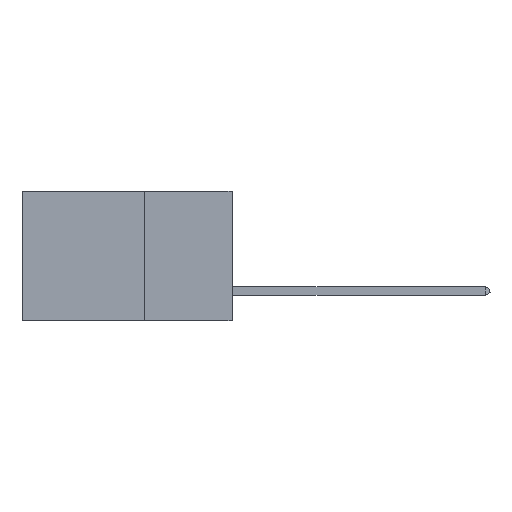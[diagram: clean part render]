
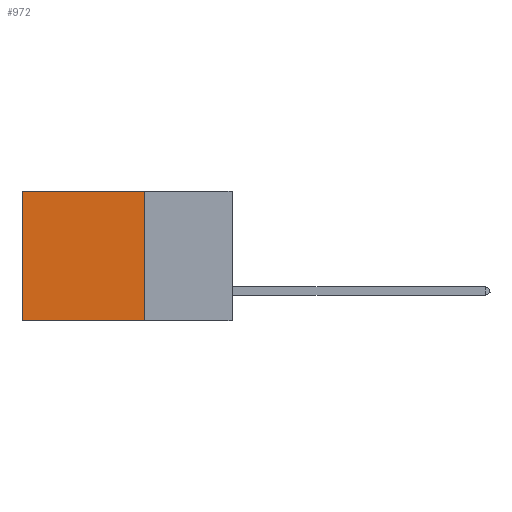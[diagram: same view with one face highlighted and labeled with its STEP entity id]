
A CAD part, left-side view. The second image highlights one B-rep face of the part: STEP entity #972.
In plain terms, the highlighted planar face has unit normal (-1, 0, 0).
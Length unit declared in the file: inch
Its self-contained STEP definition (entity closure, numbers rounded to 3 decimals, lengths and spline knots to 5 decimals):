
#972 = ADVANCED_FACE ( 'NONE', ( #11237 ), #6562, .F. ) ;
#2594 = VERTEX_POINT ( 'NONE', #11656 ) ;
#3535 = EDGE_CURVE ( 'NONE', #2594, #25100, #17388, .T. ) ;
#3725 = DIRECTION ( 'NONE',  ( 0., 1., 0. ) ) ;
#4094 = VECTOR ( 'NONE', #16937, 39.37008 ) ;
#5048 = CARTESIAN_POINT ( 'NONE',  ( 0.2875, 0.25, 0. ) ) ;
#5547 = LINE ( 'NONE', #22065, #7748 ) ;
#5821 = CARTESIAN_POINT ( 'NONE',  ( 0.2875, 0.6, 0. ) ) ;
#6021 = DIRECTION ( 'NONE',  ( 0., 1., 0. ) ) ;
#6309 = ORIENTED_EDGE ( 'NONE', *, *, #3535, .T. ) ;
#6474 = VERTEX_POINT ( 'NONE', #9506 ) ;
#6562 = PLANE ( 'NONE',  #19658 ) ;
#6997 = VECTOR ( 'NONE', #3725, 39.37008 ) ;
#7018 = DIRECTION ( 'NONE',  ( 1., 0., 0. ) ) ;
#7748 = VECTOR ( 'NONE', #6021, 39.37008 ) ;
#9506 = CARTESIAN_POINT ( 'NONE',  ( 0.2875, 0.6, -0.37 ) ) ;
#11051 = EDGE_LOOP ( 'NONE', ( #11086, #16928, #11794, #6309 ) ) ;
#11086 = ORIENTED_EDGE ( 'NONE', *, *, #21459, .T. ) ;
#11237 = FACE_OUTER_BOUND ( 'NONE', #11051, .T. ) ;
#11656 = CARTESIAN_POINT ( 'NONE',  ( 0.2875, 0.25, 0. ) ) ;
#11794 = ORIENTED_EDGE ( 'NONE', *, *, #22463, .F. ) ;
#12983 = CARTESIAN_POINT ( 'NONE',  ( 0.2875, 0.25, 0. ) ) ;
#15703 = DIRECTION ( 'NONE',  ( 0., 0., -1. ) ) ;
#15734 = LINE ( 'NONE', #5048, #4094 ) ;
#16928 = ORIENTED_EDGE ( 'NONE', *, *, #24089, .F. ) ;
#16937 = DIRECTION ( 'NONE',  ( 0., 0., -1. ) ) ;
#17365 = VECTOR ( 'NONE', #15703, 39.37008 ) ;
#17388 = LINE ( 'NONE', #25678, #6997 ) ;
#17872 = VERTEX_POINT ( 'NONE', #24602 ) ;
#19658 = AXIS2_PLACEMENT_3D ( 'NONE', #12983, #7018, #22870 ) ;
#21459 = EDGE_CURVE ( 'NONE', #25100, #6474, #22093, .T. ) ;
#22065 = CARTESIAN_POINT ( 'NONE',  ( 0.2875, 0.25, -0.37 ) ) ;
#22093 = LINE ( 'NONE', #5821, #17365 ) ;
#22463 = EDGE_CURVE ( 'NONE', #2594, #17872, #15734, .T. ) ;
#22870 = DIRECTION ( 'NONE',  ( 0., 0., -1. ) ) ;
#23224 = CARTESIAN_POINT ( 'NONE',  ( 0.2875, 0.6, 0. ) ) ;
#24089 = EDGE_CURVE ( 'NONE', #17872, #6474, #5547, .T. ) ;
#24602 = CARTESIAN_POINT ( 'NONE',  ( 0.2875, 0.25, -0.37 ) ) ;
#25100 = VERTEX_POINT ( 'NONE', #23224 ) ;
#25678 = CARTESIAN_POINT ( 'NONE',  ( 0.2875, 0.25, 0. ) ) ;
